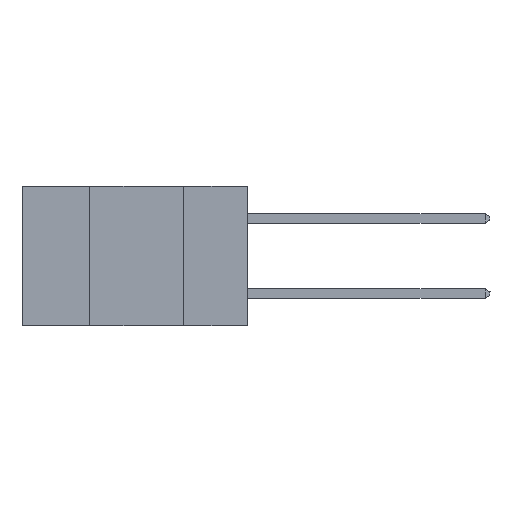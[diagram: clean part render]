
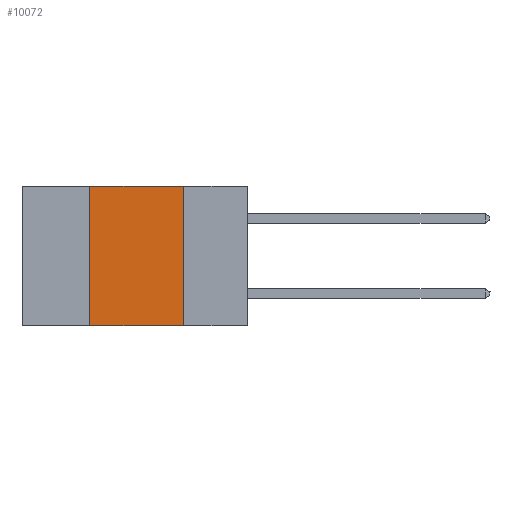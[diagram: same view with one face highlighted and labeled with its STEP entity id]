
A CAD part, left-side view. The second image highlights one B-rep face of the part: STEP entity #10072.
In plain terms, the highlighted planar face has unit normal (-1, 0, 0).
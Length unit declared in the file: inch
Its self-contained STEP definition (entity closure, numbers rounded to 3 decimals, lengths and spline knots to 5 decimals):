
#177 = CARTESIAN_POINT ( 'NONE',  ( 0., 0.17, 0. ) ) ;
#1545 = VECTOR ( 'NONE', #7752, 39.37008 ) ;
#2364 = VERTEX_POINT ( 'NONE', #14008 ) ;
#2647 = FACE_OUTER_BOUND ( 'NONE', #5859, .T. ) ;
#2949 = VECTOR ( 'NONE', #10329, 39.37008 ) ;
#3694 = VERTEX_POINT ( 'NONE', #5892 ) ;
#5859 = EDGE_LOOP ( 'NONE', ( #12271, #18998, #11860, #20253 ) ) ;
#5892 = CARTESIAN_POINT ( 'NONE',  ( 0., 0.42, 0. ) ) ;
#7037 = CARTESIAN_POINT ( 'NONE',  ( 0., 0.6, -0.37 ) ) ;
#7422 = LINE ( 'NONE', #177, #2949 ) ;
#7481 = VERTEX_POINT ( 'NONE', #19897 ) ;
#7721 = LINE ( 'NONE', #7037, #19677 ) ;
#7752 = DIRECTION ( 'NONE',  ( 0., 0., 1. ) ) ;
#8347 = DIRECTION ( 'NONE',  ( 0., -1., 0. ) ) ;
#8462 = EDGE_CURVE ( 'NONE', #3694, #21417, #16782, .T. ) ;
#8536 = PLANE ( 'NONE',  #11836 ) ;
#10072 = ADVANCED_FACE ( 'NONE', ( #2647 ), #8536, .F. ) ;
#10200 = CARTESIAN_POINT ( 'NONE',  ( 0., 0.6, 0. ) ) ;
#10329 = DIRECTION ( 'NONE',  ( 0., 0., -1. ) ) ;
#10934 = CARTESIAN_POINT ( 'NONE',  ( 0., 0.42, 0. ) ) ;
#11836 = AXIS2_PLACEMENT_3D ( 'NONE', #10200, #11850, #18307 ) ;
#11850 = DIRECTION ( 'NONE',  ( 1., 0., 0. ) ) ;
#11860 = ORIENTED_EDGE ( 'NONE', *, *, #16777, .F. ) ;
#11984 = CARTESIAN_POINT ( 'NONE',  ( 0., 0.17, 0. ) ) ;
#12271 = ORIENTED_EDGE ( 'NONE', *, *, #21395, .F. ) ;
#14008 = CARTESIAN_POINT ( 'NONE',  ( 0., 0.17, -0.37 ) ) ;
#14305 = EDGE_CURVE ( 'NONE', #7481, #2364, #7721, .T. ) ;
#14880 = CARTESIAN_POINT ( 'NONE',  ( 0., 0.6, 0. ) ) ;
#15932 = LINE ( 'NONE', #10934, #1545 ) ;
#16015 = VECTOR ( 'NONE', #8347, 39.37008 ) ;
#16777 = EDGE_CURVE ( 'NONE', #7481, #3694, #15932, .T. ) ;
#16782 = LINE ( 'NONE', #14880, #16015 ) ;
#16927 = DIRECTION ( 'NONE',  ( 0., -1., 0. ) ) ;
#18307 = DIRECTION ( 'NONE',  ( 0., 0., -1. ) ) ;
#18998 = ORIENTED_EDGE ( 'NONE', *, *, #8462, .F. ) ;
#19677 = VECTOR ( 'NONE', #16927, 39.37008 ) ;
#19897 = CARTESIAN_POINT ( 'NONE',  ( 0., 0.42, -0.37 ) ) ;
#20253 = ORIENTED_EDGE ( 'NONE', *, *, #14305, .T. ) ;
#21395 = EDGE_CURVE ( 'NONE', #21417, #2364, #7422, .T. ) ;
#21417 = VERTEX_POINT ( 'NONE', #11984 ) ;
